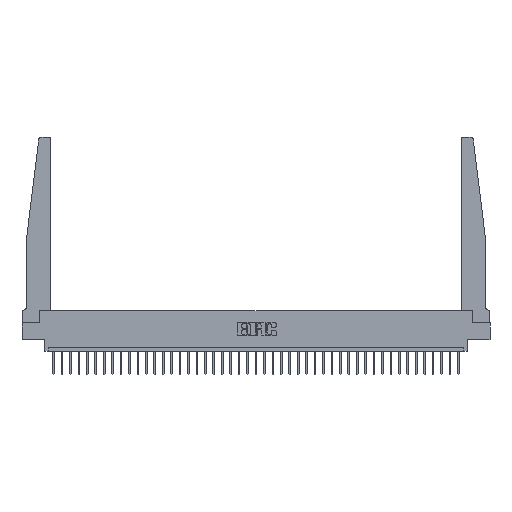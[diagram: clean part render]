
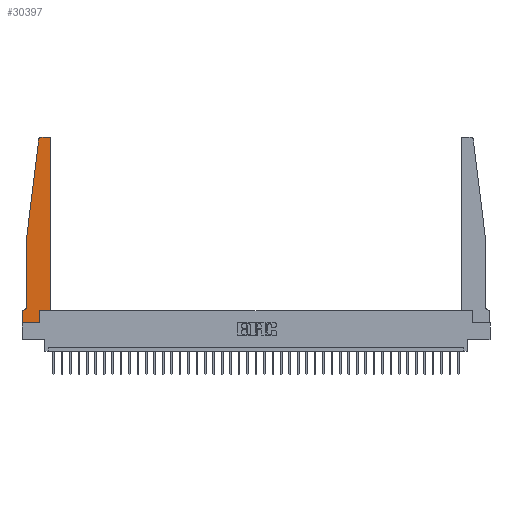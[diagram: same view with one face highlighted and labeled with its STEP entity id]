
A CAD part, top view. The second image highlights one B-rep face of the part: STEP entity #30397.
In plain terms, the highlighted planar face has unit normal (0, 0, 1).
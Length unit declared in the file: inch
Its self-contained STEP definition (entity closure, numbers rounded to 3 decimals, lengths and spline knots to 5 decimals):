
#7 = VECTOR ( 'NONE', #11220, 39.37008 ) ;
#192 = VERTEX_POINT ( 'NONE', #30077 ) ;
#453 = DIRECTION ( 'NONE',  ( 0., 1., 0. ) ) ;
#482 = LINE ( 'NONE', #10888, #7 ) ;
#639 = VECTOR ( 'NONE', #30947, 39.37008 ) ;
#647 = CARTESIAN_POINT ( 'NONE',  ( 0.2605, 0., 0.37 ) ) ;
#1401 = VECTOR ( 'NONE', #14345, 39.37008 ) ;
#1989 = EDGE_CURVE ( 'NONE', #21339, #33962, #9764, .T. ) ;
#2181 = CARTESIAN_POINT ( 'NONE',  ( 0., 0., 0.37 ) ) ;
#2262 = CARTESIAN_POINT ( 'NONE',  ( 0.015, 0.2375, 0.37 ) ) ;
#2315 = CARTESIAN_POINT ( 'NONE',  ( 0.395, 2.72, 0.37 ) ) ;
#2490 = EDGE_LOOP ( 'NONE', ( #19024, #9183, #9975, #22958, #6858, #2735, #18670, #7376, #6298, #30567, #13905, #15250 ) ) ;
#2735 = ORIENTED_EDGE ( 'NONE', *, *, #17759, .T. ) ;
#3003 = VERTEX_POINT ( 'NONE', #26273 ) ;
#3359 = DIRECTION ( 'NONE',  ( 0., -1., 0. ) ) ;
#4504 = PLANE ( 'NONE',  #25647 ) ;
#4570 = DIRECTION ( 'NONE',  ( 0., 0., 1. ) ) ;
#5054 = VERTEX_POINT ( 'NONE', #30132 ) ;
#5069 = DIRECTION ( 'NONE',  ( -1., 0., 0. ) ) ;
#5560 = CIRCLE ( 'NONE', #25203, 0.05 ) ;
#5718 = LINE ( 'NONE', #11014, #23186 ) ;
#5846 = VERTEX_POINT ( 'NONE', #10648 ) ;
#5847 = DIRECTION ( 'NONE',  ( 1., 0., 0. ) ) ;
#6209 = VECTOR ( 'NONE', #25234, 39.37008 ) ;
#6298 = ORIENTED_EDGE ( 'NONE', *, *, #20135, .T. ) ;
#6423 = VERTEX_POINT ( 'NONE', #30990 ) ;
#6785 = CARTESIAN_POINT ( 'NONE',  ( 0.425, 2.72, 0.37 ) ) ;
#6800 = CIRCLE ( 'NONE', #22507, 0.03 ) ;
#6858 = ORIENTED_EDGE ( 'NONE', *, *, #11871, .T. ) ;
#7163 = CARTESIAN_POINT ( 'NONE',  ( 0.065, 0.1875, 0.37 ) ) ;
#7376 = ORIENTED_EDGE ( 'NONE', *, *, #32727, .T. ) ;
#7489 = LINE ( 'NONE', #12763, #31459 ) ;
#7501 = EDGE_CURVE ( 'NONE', #192, #33459, #17084, .T. ) ;
#7785 = EDGE_CURVE ( 'NONE', #5054, #21339, #26625, .T. ) ;
#8606 = CARTESIAN_POINT ( 'NONE',  ( 0.065, 1.25, 0.37 ) ) ;
#9183 = ORIENTED_EDGE ( 'NONE', *, *, #7501, .T. ) ;
#9764 = LINE ( 'NONE', #14484, #6209 ) ;
#9856 = VECTOR ( 'NONE', #5847, 39.37008 ) ;
#9975 = ORIENTED_EDGE ( 'NONE', *, *, #22659, .T. ) ;
#10180 = VECTOR ( 'NONE', #22801, 39.37008 ) ;
#10648 = CARTESIAN_POINT ( 'NONE',  ( 0.065, 0.2375, 0.37 ) ) ;
#10888 = CARTESIAN_POINT ( 'NONE',  ( 0.065, 1.25, 0.37 ) ) ;
#10957 = VERTEX_POINT ( 'NONE', #647 ) ;
#10973 = CARTESIAN_POINT ( 'NONE',  ( 0.425, 0.18, 0.37 ) ) ;
#11014 = CARTESIAN_POINT ( 'NONE',  ( 0.2605, 0.18, 0.37 ) ) ;
#11220 = DIRECTION ( 'NONE',  ( 0., -1., 0. ) ) ;
#11793 = CARTESIAN_POINT ( 'NONE',  ( 0., 0., 0.37 ) ) ;
#11868 = CARTESIAN_POINT ( 'NONE',  ( 0.27653, 2.72, 0.37 ) ) ;
#11871 = EDGE_CURVE ( 'NONE', #5846, #6423, #5560, .T. ) ;
#11954 = LINE ( 'NONE', #14544, #10180 ) ;
#12266 = DIRECTION ( 'NONE',  ( 0., 0., 1. ) ) ;
#12329 = VERTEX_POINT ( 'NONE', #17632 ) ;
#12466 = DIRECTION ( 'NONE',  ( 0., 0., -1. ) ) ;
#12763 = CARTESIAN_POINT ( 'NONE',  ( 0., 0., 0.37 ) ) ;
#13905 = ORIENTED_EDGE ( 'NONE', *, *, #1989, .T. ) ;
#14345 = DIRECTION ( 'NONE',  ( -0.122, -0.992, 0. ) ) ;
#14484 = CARTESIAN_POINT ( 'NONE',  ( 0.425, 0.18, 0.37 ) ) ;
#14544 = CARTESIAN_POINT ( 'NONE',  ( 0.25, 2.75, 0.37 ) ) ;
#14690 = DIRECTION ( 'NONE',  ( 1., 0., 0. ) ) ;
#15250 = ORIENTED_EDGE ( 'NONE', *, *, #23391, .T. ) ;
#15274 = DIRECTION ( 'NONE',  ( 1., 0., 0. ) ) ;
#15872 = VECTOR ( 'NONE', #3359, 39.37008 ) ;
#17084 = CIRCLE ( 'NONE', #26129, 0.03 ) ;
#17632 = CARTESIAN_POINT ( 'NONE',  ( 0.395, 2.75, 0.37 ) ) ;
#17759 = EDGE_CURVE ( 'NONE', #6423, #3003, #25615, .T. ) ;
#17857 = CARTESIAN_POINT ( 'NONE',  ( 0.24675, 2.72367, 0.37 ) ) ;
#18343 = DIRECTION ( 'NONE',  ( 1., 0., 0. ) ) ;
#18670 = ORIENTED_EDGE ( 'NONE', *, *, #21116, .T. ) ;
#19024 = ORIENTED_EDGE ( 'NONE', *, *, #23618, .T. ) ;
#19452 = LINE ( 'NONE', #8606, #1401 ) ;
#19922 = DIRECTION ( 'NONE',  ( 0., 0., 1. ) ) ;
#20135 = EDGE_CURVE ( 'NONE', #10957, #5054, #5718, .T. ) ;
#20479 = CARTESIAN_POINT ( 'NONE',  ( 0., 0.1875, 0.37 ) ) ;
#21116 = EDGE_CURVE ( 'NONE', #3003, #25840, #21960, .T. ) ;
#21222 = CARTESIAN_POINT ( 'NONE',  ( 0.425, 0.18, 0.37 ) ) ;
#21339 = VERTEX_POINT ( 'NONE', #21222 ) ;
#21960 = LINE ( 'NONE', #11793, #15872 ) ;
#22507 = AXIS2_PLACEMENT_3D ( 'NONE', #2315, #4570, #15274 ) ;
#22659 = EDGE_CURVE ( 'NONE', #33459, #23370, #19452, .T. ) ;
#22801 = DIRECTION ( 'NONE',  ( -1., 0., 0. ) ) ;
#22958 = ORIENTED_EDGE ( 'NONE', *, *, #33791, .T. ) ;
#23186 = VECTOR ( 'NONE', #453, 39.37008 ) ;
#23370 = VERTEX_POINT ( 'NONE', #23546 ) ;
#23391 = EDGE_CURVE ( 'NONE', #33962, #12329, #6800, .T. ) ;
#23546 = CARTESIAN_POINT ( 'NONE',  ( 0.065, 1.25, 0.37 ) ) ;
#23618 = EDGE_CURVE ( 'NONE', #12329, #192, #11954, .T. ) ;
#25203 = AXIS2_PLACEMENT_3D ( 'NONE', #2262, #12466, #5069 ) ;
#25234 = DIRECTION ( 'NONE',  ( 0., 1., 0. ) ) ;
#25615 = LINE ( 'NONE', #7163, #639 ) ;
#25647 = AXIS2_PLACEMENT_3D ( 'NONE', #20479, #12266, #14690 ) ;
#25840 = VERTEX_POINT ( 'NONE', #2181 ) ;
#26129 = AXIS2_PLACEMENT_3D ( 'NONE', #11868, #19922, #30709 ) ;
#26273 = CARTESIAN_POINT ( 'NONE',  ( 0., 0.1875, 0.37 ) ) ;
#26625 = LINE ( 'NONE', #10973, #9856 ) ;
#28126 = FACE_OUTER_BOUND ( 'NONE', #2490, .T. ) ;
#30077 = CARTESIAN_POINT ( 'NONE',  ( 0.27653, 2.75, 0.37 ) ) ;
#30132 = CARTESIAN_POINT ( 'NONE',  ( 0.2605, 0.18, 0.37 ) ) ;
#30397 = ADVANCED_FACE ( 'NONE', ( #28126 ), #4504, .T. ) ;
#30567 = ORIENTED_EDGE ( 'NONE', *, *, #7785, .T. ) ;
#30709 = DIRECTION ( 'NONE',  ( 1., 0., 0. ) ) ;
#30947 = DIRECTION ( 'NONE',  ( -1., 0., 0. ) ) ;
#30990 = CARTESIAN_POINT ( 'NONE',  ( 0.015, 0.1875, 0.37 ) ) ;
#31459 = VECTOR ( 'NONE', #18343, 39.37008 ) ;
#32727 = EDGE_CURVE ( 'NONE', #25840, #10957, #7489, .T. ) ;
#33459 = VERTEX_POINT ( 'NONE', #17857 ) ;
#33791 = EDGE_CURVE ( 'NONE', #23370, #5846, #482, .T. ) ;
#33962 = VERTEX_POINT ( 'NONE', #6785 ) ;
